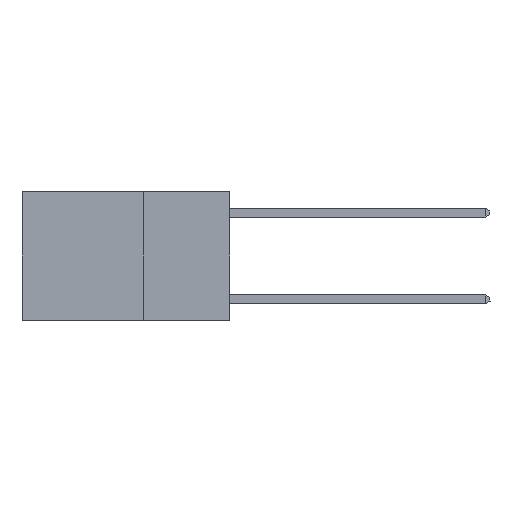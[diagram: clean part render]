
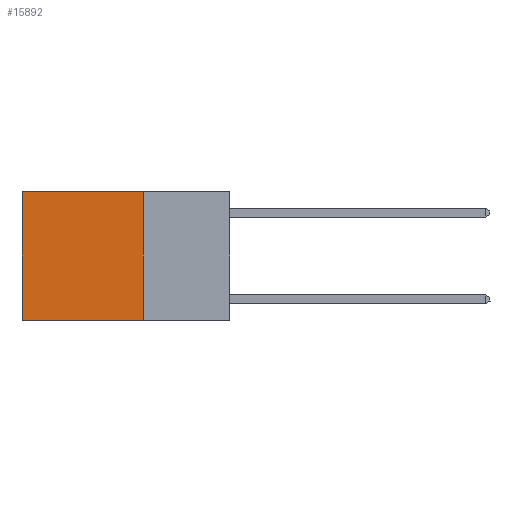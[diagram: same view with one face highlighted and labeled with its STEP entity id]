
A CAD part, left-side view. The second image highlights one B-rep face of the part: STEP entity #15892.
In plain terms, the highlighted planar face has unit normal (-1, 0, 0).
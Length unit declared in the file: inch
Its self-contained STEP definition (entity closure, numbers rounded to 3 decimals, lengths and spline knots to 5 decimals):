
#514 = CARTESIAN_POINT ( 'NONE',  ( 0.2625, 0.25, 0. ) ) ;
#643 = ORIENTED_EDGE ( 'NONE', *, *, #1367, .T. ) ;
#933 = CARTESIAN_POINT ( 'NONE',  ( 0.2625, 0.25, 0. ) ) ;
#1367 = EDGE_CURVE ( 'NONE', #21415, #10550, #16547, .T. ) ;
#1893 = VECTOR ( 'NONE', #29638, 39.37008 ) ;
#2524 = CARTESIAN_POINT ( 'NONE',  ( 0.2625, 0.25, 0. ) ) ;
#3078 = VECTOR ( 'NONE', #12659, 39.37008 ) ;
#3258 = ORIENTED_EDGE ( 'NONE', *, *, #7249, .T. ) ;
#3354 = CARTESIAN_POINT ( 'NONE',  ( 0.2625, 0.6, 0. ) ) ;
#5607 = CARTESIAN_POINT ( 'NONE',  ( 0.2625, 0.6, -0.37 ) ) ;
#7249 = EDGE_CURVE ( 'NONE', #10550, #19107, #26606, .T. ) ;
#7591 = VERTEX_POINT ( 'NONE', #14065 ) ;
#8157 = CARTESIAN_POINT ( 'NONE',  ( 0.2625, 0.6, 0. ) ) ;
#10550 = VERTEX_POINT ( 'NONE', #8157 ) ;
#12468 = AXIS2_PLACEMENT_3D ( 'NONE', #514, #29439, #15017 ) ;
#12505 = CARTESIAN_POINT ( 'NONE',  ( 0.2625, 0.25, 0. ) ) ;
#12659 = DIRECTION ( 'NONE',  ( 0., 1., 0. ) ) ;
#14065 = CARTESIAN_POINT ( 'NONE',  ( 0.2625, 0.25, -0.37 ) ) ;
#14843 = DIRECTION ( 'NONE',  ( 0., 0., -1. ) ) ;
#15017 = DIRECTION ( 'NONE',  ( 0., 0., -1. ) ) ;
#15411 = ORIENTED_EDGE ( 'NONE', *, *, #22237, .F. ) ;
#15725 = CARTESIAN_POINT ( 'NONE',  ( 0.2625, 0.25, -0.37 ) ) ;
#15892 = ADVANCED_FACE ( 'NONE', ( #28694 ), #27020, .F. ) ;
#16547 = LINE ( 'NONE', #2524, #3078 ) ;
#16570 = EDGE_LOOP ( 'NONE', ( #3258, #15411, #20889, #643 ) ) ;
#17180 = LINE ( 'NONE', #15725, #22836 ) ;
#19107 = VERTEX_POINT ( 'NONE', #5607 ) ;
#20597 = DIRECTION ( 'NONE',  ( 0., 1., 0. ) ) ;
#20889 = ORIENTED_EDGE ( 'NONE', *, *, #22680, .F. ) ;
#21415 = VERTEX_POINT ( 'NONE', #933 ) ;
#22237 = EDGE_CURVE ( 'NONE', #7591, #19107, #17180, .T. ) ;
#22680 = EDGE_CURVE ( 'NONE', #21415, #7591, #29944, .T. ) ;
#22804 = VECTOR ( 'NONE', #14843, 39.37008 ) ;
#22836 = VECTOR ( 'NONE', #20597, 39.37008 ) ;
#26606 = LINE ( 'NONE', #3354, #1893 ) ;
#27020 = PLANE ( 'NONE',  #12468 ) ;
#28694 = FACE_OUTER_BOUND ( 'NONE', #16570, .T. ) ;
#29439 = DIRECTION ( 'NONE',  ( 1., 0., 0. ) ) ;
#29638 = DIRECTION ( 'NONE',  ( 0., 0., -1. ) ) ;
#29944 = LINE ( 'NONE', #12505, #22804 ) ;
